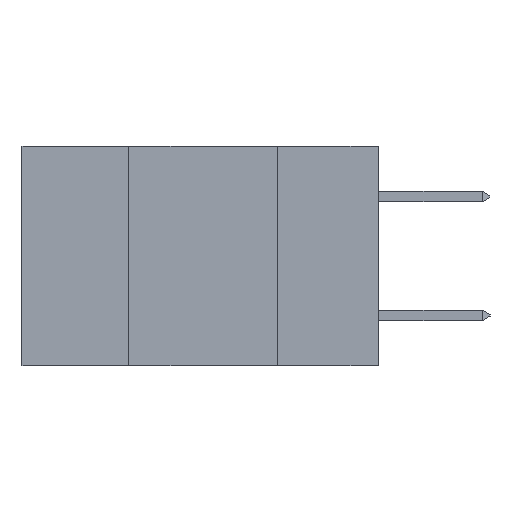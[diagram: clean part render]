
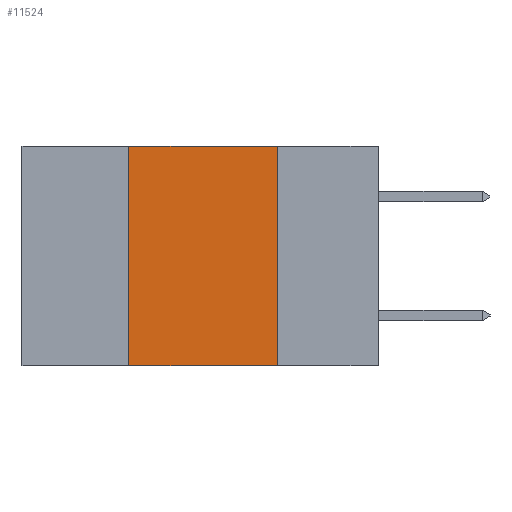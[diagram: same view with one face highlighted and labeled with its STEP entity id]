
A CAD part, left-side view. The second image highlights one B-rep face of the part: STEP entity #11524.
In plain terms, the highlighted planar face has unit normal (-1, 0, 0).
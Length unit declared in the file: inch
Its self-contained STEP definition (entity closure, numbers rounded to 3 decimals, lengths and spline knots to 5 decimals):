
#578 = EDGE_CURVE ( 'NONE', #1103, #14443, #10126, .T. ) ;
#1103 = VERTEX_POINT ( 'NONE', #14003 ) ;
#1230 = PLANE ( 'NONE',  #5807 ) ;
#1884 = DIRECTION ( 'NONE',  ( 0., 0., -1. ) ) ;
#2052 = ORIENTED_EDGE ( 'NONE', *, *, #7454, .F. ) ;
#3035 = VECTOR ( 'NONE', #11909, 39.37008 ) ;
#3306 = VECTOR ( 'NONE', #6386, 39.37008 ) ;
#3631 = CARTESIAN_POINT ( 'NONE',  ( 0., 0.6, -0.37 ) ) ;
#4060 = DIRECTION ( 'NONE',  ( 1., 0., 0. ) ) ;
#4667 = EDGE_CURVE ( 'NONE', #1103, #7881, #10402, .T. ) ;
#5089 = CARTESIAN_POINT ( 'NONE',  ( 0., 0.17, -0.37 ) ) ;
#5224 = ORIENTED_EDGE ( 'NONE', *, *, #578, .T. ) ;
#5807 = AXIS2_PLACEMENT_3D ( 'NONE', #11996, #4060, #13388 ) ;
#6386 = DIRECTION ( 'NONE',  ( 0., -1., 0. ) ) ;
#6408 = LINE ( 'NONE', #14417, #3306 ) ;
#6839 = VECTOR ( 'NONE', #7392, 39.37008 ) ;
#7392 = DIRECTION ( 'NONE',  ( 0., 0., 1. ) ) ;
#7454 = EDGE_CURVE ( 'NONE', #7881, #8579, #6408, .T. ) ;
#7742 = CARTESIAN_POINT ( 'NONE',  ( 0., 0.42, -0.37 ) ) ;
#7881 = VERTEX_POINT ( 'NONE', #15258 ) ;
#8579 = VERTEX_POINT ( 'NONE', #15573 ) ;
#9137 = ORIENTED_EDGE ( 'NONE', *, *, #4667, .F. ) ;
#10126 = LINE ( 'NONE', #3631, #3035 ) ;
#10402 = LINE ( 'NONE', #7742, #6839 ) ;
#10920 = VECTOR ( 'NONE', #1884, 39.37008 ) ;
#11355 = LINE ( 'NONE', #12639, #10920 ) ;
#11524 = ADVANCED_FACE ( 'NONE', ( #11546 ), #1230, .F. ) ;
#11546 = FACE_OUTER_BOUND ( 'NONE', #17086, .T. ) ;
#11909 = DIRECTION ( 'NONE',  ( 0., -1., 0. ) ) ;
#11996 = CARTESIAN_POINT ( 'NONE',  ( 0., 0.6, 0. ) ) ;
#12639 = CARTESIAN_POINT ( 'NONE',  ( 0., 0.17, -0.37 ) ) ;
#13241 = ORIENTED_EDGE ( 'NONE', *, *, #14923, .F. ) ;
#13388 = DIRECTION ( 'NONE',  ( 0., 0., -1. ) ) ;
#14003 = CARTESIAN_POINT ( 'NONE',  ( 0., 0.42, -0.37 ) ) ;
#14417 = CARTESIAN_POINT ( 'NONE',  ( 0., 0.6, 0. ) ) ;
#14443 = VERTEX_POINT ( 'NONE', #5089 ) ;
#14923 = EDGE_CURVE ( 'NONE', #8579, #14443, #11355, .T. ) ;
#15258 = CARTESIAN_POINT ( 'NONE',  ( 0., 0.42, 0. ) ) ;
#15573 = CARTESIAN_POINT ( 'NONE',  ( 0., 0.17, 0. ) ) ;
#17086 = EDGE_LOOP ( 'NONE', ( #13241, #2052, #9137, #5224 ) ) ;
